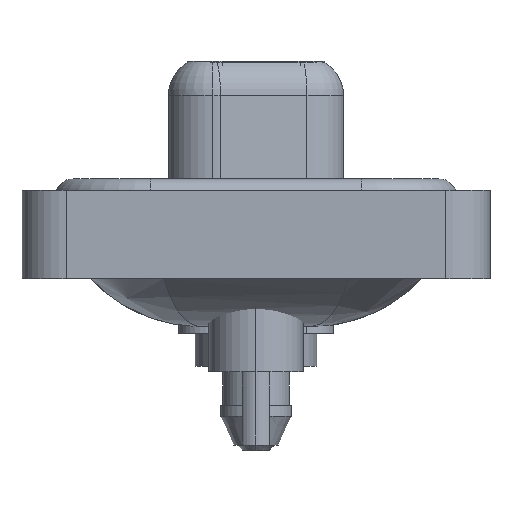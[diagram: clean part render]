
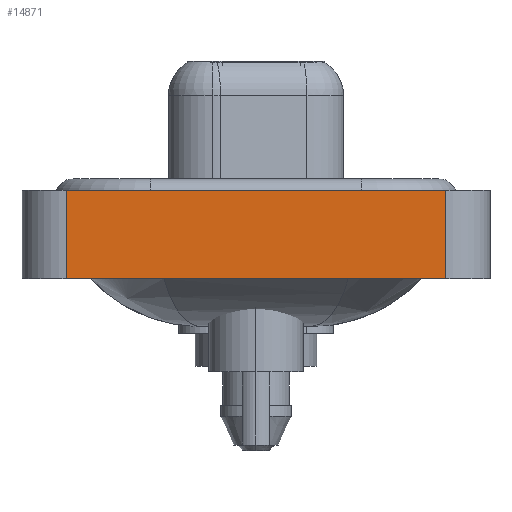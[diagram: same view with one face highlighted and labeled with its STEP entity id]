
A CAD part, left-side view. The second image highlights one B-rep face of the part: STEP entity #14871.
In plain terms, the highlighted planar face has unit normal (-1, 0, 0).
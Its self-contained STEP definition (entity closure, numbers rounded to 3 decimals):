
#20 = PLANE ( 'NONE',  #11393 ) ;
#178 = CARTESIAN_POINT ( 'NONE',  ( -7.3, -8.55, 0.4 ) ) ;
#1430 = VERTEX_POINT ( 'NONE', #15849 ) ;
#1726 = CARTESIAN_POINT ( 'NONE',  ( -7.3, -8.55, -3.6 ) ) ;
#2235 = VERTEX_POINT ( 'NONE', #178 ) ;
#2514 = LINE ( 'NONE', #10628, #2612 ) ;
#2612 = VECTOR ( 'NONE', #10383, 1000. ) ;
#2845 = VECTOR ( 'NONE', #4494, 1000. ) ;
#2987 = DIRECTION ( 'NONE',  ( 0., 0., 1. ) ) ;
#3333 = EDGE_CURVE ( 'NONE', #1430, #11498, #2514, .T. ) ;
#3764 = CARTESIAN_POINT ( 'NONE',  ( -7.3, -8.55, -3.6 ) ) ;
#3976 = DIRECTION ( 'NONE',  ( 0., 0., 1. ) ) ;
#4023 = FACE_OUTER_BOUND ( 'NONE', #8616, .T. ) ;
#4254 = EDGE_CURVE ( 'NONE', #11498, #2235, #5373, .T. ) ;
#4360 = VECTOR ( 'NONE', #2987, 1000. ) ;
#4494 = DIRECTION ( 'NONE',  ( 0., -1., 0. ) ) ;
#5361 = VECTOR ( 'NONE', #3976, 1000. ) ;
#5373 = LINE ( 'NONE', #1726, #4360 ) ;
#5598 = ORIENTED_EDGE ( 'NONE', *, *, #5932, .F. ) ;
#5932 = EDGE_CURVE ( 'NONE', #1430, #13172, #16728, .T. ) ;
#6333 = ORIENTED_EDGE ( 'NONE', *, *, #4254, .T. ) ;
#7040 = ORIENTED_EDGE ( 'NONE', *, *, #16050, .F. ) ;
#8098 = ORIENTED_EDGE ( 'NONE', *, *, #3333, .T. ) ;
#8616 = EDGE_LOOP ( 'NONE', ( #6333, #7040, #5598, #8098 ) ) ;
#8668 = CARTESIAN_POINT ( 'NONE',  ( -7.3, -8.55, 0.4 ) ) ;
#10383 = DIRECTION ( 'NONE',  ( 0., -1., 0. ) ) ;
#10628 = CARTESIAN_POINT ( 'NONE',  ( -7.3, -8.55, -3.6 ) ) ;
#11393 = AXIS2_PLACEMENT_3D ( 'NONE', #11873, #16779, #12886 ) ;
#11498 = VERTEX_POINT ( 'NONE', #3764 ) ;
#11873 = CARTESIAN_POINT ( 'NONE',  ( -7.3, -8.55, -3.6 ) ) ;
#12886 = DIRECTION ( 'NONE',  ( 0., 0., 1. ) ) ;
#12959 = CARTESIAN_POINT ( 'NONE',  ( -7.3, 8.55, 0.4 ) ) ;
#13172 = VERTEX_POINT ( 'NONE', #12959 ) ;
#13949 = CARTESIAN_POINT ( 'NONE',  ( -7.3, 8.55, -3.6 ) ) ;
#14871 = ADVANCED_FACE ( 'NONE', ( #4023 ), #20, .T. ) ;
#15849 = CARTESIAN_POINT ( 'NONE',  ( -7.3, 8.55, -3.6 ) ) ;
#16050 = EDGE_CURVE ( 'NONE', #13172, #2235, #16394, .T. ) ;
#16394 = LINE ( 'NONE', #8668, #2845 ) ;
#16728 = LINE ( 'NONE', #13949, #5361 ) ;
#16779 = DIRECTION ( 'NONE',  ( -1., 0., 0. ) ) ;
